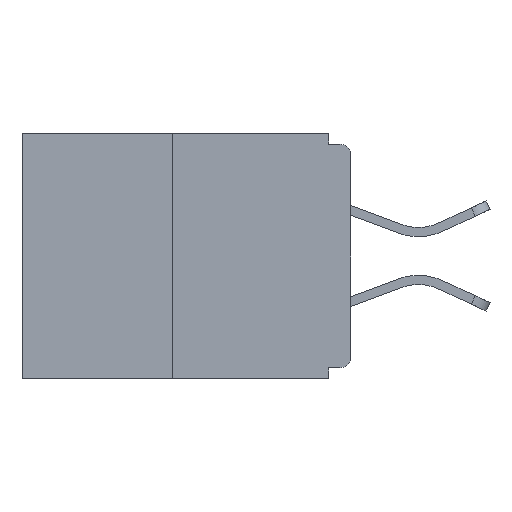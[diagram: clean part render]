
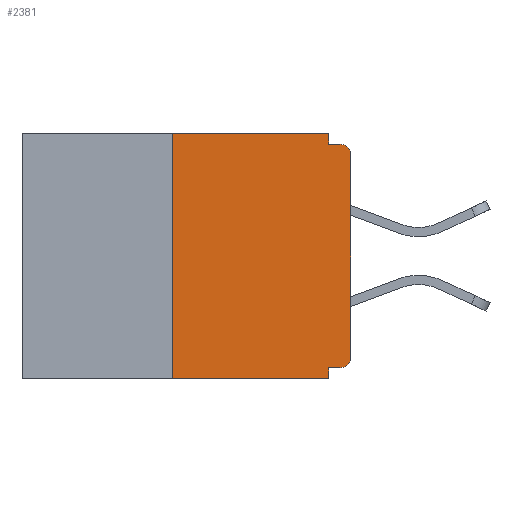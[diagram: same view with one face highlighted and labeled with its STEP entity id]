
A CAD part, left-side view. The second image highlights one B-rep face of the part: STEP entity #2381.
In plain terms, the highlighted planar face has unit normal (-1, 0, 0).
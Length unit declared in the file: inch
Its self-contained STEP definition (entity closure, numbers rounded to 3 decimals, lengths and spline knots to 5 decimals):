
#190 = ORIENTED_EDGE ( 'NONE', *, *, #3893, .T. ) ;
#588 = VECTOR ( 'NONE', #1454, 39.37008 ) ;
#645 = DIRECTION ( 'NONE',  ( 0., 0., -1. ) ) ;
#806 = VERTEX_POINT ( 'NONE', #9260 ) ;
#1005 = LINE ( 'NONE', #10246, #9034 ) ;
#1454 = DIRECTION ( 'NONE',  ( 0., 0., 1. ) ) ;
#1505 = VECTOR ( 'NONE', #3634, 39.37008 ) ;
#1560 = VERTEX_POINT ( 'NONE', #5880 ) ;
#1692 = LINE ( 'NONE', #4531, #8426 ) ;
#1825 = CARTESIAN_POINT ( 'NONE',  ( 0., 0.031, -0.015 ) ) ;
#2125 = VECTOR ( 'NONE', #13125, 39.37008 ) ;
#2356 = ORIENTED_EDGE ( 'NONE', *, *, #7431, .F. ) ;
#2381 = ADVANCED_FACE ( 'NONE', ( #12846 ), #10893, .F. ) ;
#2460 = VERTEX_POINT ( 'NONE', #12008 ) ;
#2865 = CARTESIAN_POINT ( 'NONE',  ( 0., 0., -0.313 ) ) ;
#3016 = EDGE_CURVE ( 'NONE', #10406, #9314, #11310, .T. ) ;
#3017 = CARTESIAN_POINT ( 'NONE',  ( 0., 0.015, -0.015 ) ) ;
#3064 = ORIENTED_EDGE ( 'NONE', *, *, #11595, .F. ) ;
#3316 = ORIENTED_EDGE ( 'NONE', *, *, #3016, .F. ) ;
#3557 = DIRECTION ( 'NONE',  ( 0., -1., 0. ) ) ;
#3634 = DIRECTION ( 'NONE',  ( 0., 0., -1. ) ) ;
#3776 = VECTOR ( 'NONE', #3557, 39.37008 ) ;
#3893 = EDGE_CURVE ( 'NONE', #4294, #1560, #1692, .T. ) ;
#4294 = VERTEX_POINT ( 'NONE', #9167 ) ;
#4310 = LINE ( 'NONE', #5969, #11677 ) ;
#4471 = CARTESIAN_POINT ( 'NONE',  ( 0., 0.031, 0. ) ) ;
#4531 = CARTESIAN_POINT ( 'NONE',  ( 0., 0.46, -0.343 ) ) ;
#4569 = LINE ( 'NONE', #6615, #3776 ) ;
#4600 = DIRECTION ( 'NONE',  ( 0., -1., 0. ) ) ;
#4642 = DIRECTION ( 'NONE',  ( -1., 0., 0. ) ) ;
#4739 = EDGE_LOOP ( 'NONE', ( #3316, #5808, #190, #8767, #2356, #11226, #4848, #7424, #3064, #8014 ) ) ;
#4765 = DIRECTION ( 'NONE',  ( 0., 0., -1. ) ) ;
#4848 = ORIENTED_EDGE ( 'NONE', *, *, #11240, .T. ) ;
#5167 = EDGE_CURVE ( 'NONE', #4294, #10406, #5818, .T. ) ;
#5619 = EDGE_CURVE ( 'NONE', #2460, #1560, #1005, .T. ) ;
#5808 = ORIENTED_EDGE ( 'NONE', *, *, #5167, .F. ) ;
#5818 = LINE ( 'NONE', #11184, #2125 ) ;
#5880 = CARTESIAN_POINT ( 'NONE',  ( 0., 0.031, -0.343 ) ) ;
#5884 = CARTESIAN_POINT ( 'NONE',  ( 0., 0.015, -0.328 ) ) ;
#5969 = CARTESIAN_POINT ( 'NONE',  ( 0., 0., -0.328 ) ) ;
#6241 = VERTEX_POINT ( 'NONE', #5884 ) ;
#6509 = EDGE_CURVE ( 'NONE', #6241, #8522, #6571, .T. ) ;
#6566 = CARTESIAN_POINT ( 'NONE',  ( 0., 0.46, 0. ) ) ;
#6571 = CIRCLE ( 'NONE', #13176, 0.015 ) ;
#6615 = CARTESIAN_POINT ( 'NONE',  ( 0., 0., -0.015 ) ) ;
#6655 = DIRECTION ( 'NONE',  ( 1., 0., 0. ) ) ;
#6793 = CIRCLE ( 'NONE', #11529, 0.015 ) ;
#7319 = AXIS2_PLACEMENT_3D ( 'NONE', #8733, #6655, #4765 ) ;
#7324 = VERTEX_POINT ( 'NONE', #1825 ) ;
#7424 = ORIENTED_EDGE ( 'NONE', *, *, #11570, .T. ) ;
#7431 = EDGE_CURVE ( 'NONE', #6241, #2460, #4310, .T. ) ;
#7516 = CARTESIAN_POINT ( 'NONE',  ( 0., 0., 0. ) ) ;
#7724 = CARTESIAN_POINT ( 'NONE',  ( 0., 0.015, -0.313 ) ) ;
#8014 = ORIENTED_EDGE ( 'NONE', *, *, #12262, .F. ) ;
#8214 = DIRECTION ( 'NONE',  ( 0., 0., -1. ) ) ;
#8264 = VERTEX_POINT ( 'NONE', #3017 ) ;
#8426 = VECTOR ( 'NONE', #11815, 39.37008 ) ;
#8522 = VERTEX_POINT ( 'NONE', #2865 ) ;
#8535 = CARTESIAN_POINT ( 'NONE',  ( 0., 0.25, 0. ) ) ;
#8696 = DIRECTION ( 'NONE',  ( 0., 0., -1. ) ) ;
#8733 = CARTESIAN_POINT ( 'NONE',  ( 0., 0.46, 0. ) ) ;
#8767 = ORIENTED_EDGE ( 'NONE', *, *, #5619, .F. ) ;
#9034 = VECTOR ( 'NONE', #8214, 39.37008 ) ;
#9167 = CARTESIAN_POINT ( 'NONE',  ( 0., 0.25, -0.343 ) ) ;
#9260 = CARTESIAN_POINT ( 'NONE',  ( 0., 0., -0.03 ) ) ;
#9314 = VERTEX_POINT ( 'NONE', #4471 ) ;
#9355 = CARTESIAN_POINT ( 'NONE',  ( 0., 0.031, 0. ) ) ;
#9846 = LINE ( 'NONE', #9355, #1505 ) ;
#10246 = CARTESIAN_POINT ( 'NONE',  ( 0., 0.031, -0.343 ) ) ;
#10406 = VERTEX_POINT ( 'NONE', #8535 ) ;
#10693 = DIRECTION ( 'NONE',  ( -1., 0., 0. ) ) ;
#10893 = PLANE ( 'NONE',  #7319 ) ;
#11184 = CARTESIAN_POINT ( 'NONE',  ( 0., 0.25, 0. ) ) ;
#11226 = ORIENTED_EDGE ( 'NONE', *, *, #6509, .T. ) ;
#11240 = EDGE_CURVE ( 'NONE', #8522, #806, #12898, .T. ) ;
#11310 = LINE ( 'NONE', #6566, #12273 ) ;
#11529 = AXIS2_PLACEMENT_3D ( 'NONE', #12716, #10693, #8696 ) ;
#11570 = EDGE_CURVE ( 'NONE', #806, #8264, #6793, .T. ) ;
#11595 = EDGE_CURVE ( 'NONE', #7324, #8264, #4569, .T. ) ;
#11677 = VECTOR ( 'NONE', #12281, 39.37008 ) ;
#11815 = DIRECTION ( 'NONE',  ( 0., -1., 0. ) ) ;
#12008 = CARTESIAN_POINT ( 'NONE',  ( 0., 0.031, -0.328 ) ) ;
#12262 = EDGE_CURVE ( 'NONE', #9314, #7324, #9846, .T. ) ;
#12273 = VECTOR ( 'NONE', #4600, 39.37008 ) ;
#12281 = DIRECTION ( 'NONE',  ( 0., 1., 0. ) ) ;
#12716 = CARTESIAN_POINT ( 'NONE',  ( 0., 0.015, -0.03 ) ) ;
#12846 = FACE_OUTER_BOUND ( 'NONE', #4739, .T. ) ;
#12898 = LINE ( 'NONE', #7516, #588 ) ;
#13125 = DIRECTION ( 'NONE',  ( 0., 0., 1. ) ) ;
#13176 = AXIS2_PLACEMENT_3D ( 'NONE', #7724, #4642, #645 ) ;
